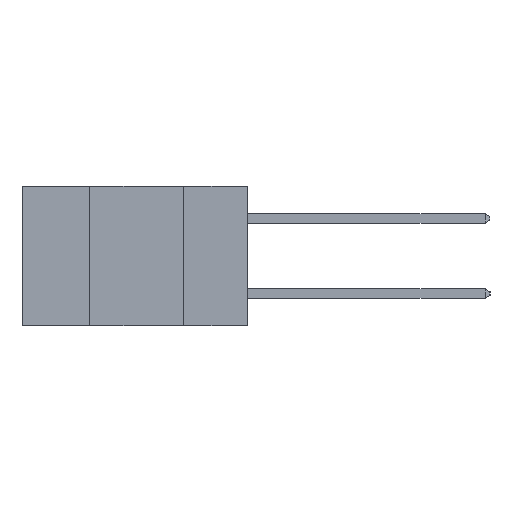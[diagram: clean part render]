
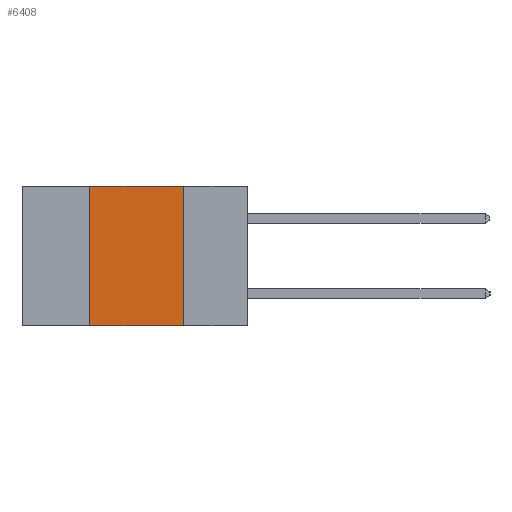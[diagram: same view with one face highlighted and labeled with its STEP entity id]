
A CAD part, left-side view. The second image highlights one B-rep face of the part: STEP entity #6408.
In plain terms, the highlighted planar face has unit normal (-1, 0, 0).
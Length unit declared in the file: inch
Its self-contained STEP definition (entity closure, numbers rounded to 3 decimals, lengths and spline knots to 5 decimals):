
#163 = DIRECTION ( 'NONE',  ( 0., -1., 0. ) ) ;
#276 = CARTESIAN_POINT ( 'NONE',  ( 0., 0.6, 0. ) ) ;
#285 = ORIENTED_EDGE ( 'NONE', *, *, #1232, .F. ) ;
#347 = VECTOR ( 'NONE', #7281, 39.37008 ) ;
#622 = DIRECTION ( 'NONE',  ( 0., 0., 1. ) ) ;
#681 = VERTEX_POINT ( 'NONE', #9778 ) ;
#891 = EDGE_LOOP ( 'NONE', ( #9026, #285, #3984, #10460 ) ) ;
#956 = LINE ( 'NONE', #11205, #10092 ) ;
#1057 = CARTESIAN_POINT ( 'NONE',  ( 0., 0.17, -0.37 ) ) ;
#1232 = EDGE_CURVE ( 'NONE', #3908, #3191, #4190, .T. ) ;
#1234 = FACE_OUTER_BOUND ( 'NONE', #891, .T. ) ;
#1329 = VERTEX_POINT ( 'NONE', #2816 ) ;
#1766 = DIRECTION ( 'NONE',  ( 0., 0., -1. ) ) ;
#2512 = EDGE_CURVE ( 'NONE', #3191, #681, #8621, .T. ) ;
#2515 = LINE ( 'NONE', #3765, #6845 ) ;
#2647 = EDGE_CURVE ( 'NONE', #1329, #681, #2515, .T. ) ;
#2704 = CARTESIAN_POINT ( 'NONE',  ( 0., 0.6, 0. ) ) ;
#2816 = CARTESIAN_POINT ( 'NONE',  ( 0., 0.42, -0.37 ) ) ;
#2960 = CARTESIAN_POINT ( 'NONE',  ( 0., 0.17, 0. ) ) ;
#3191 = VERTEX_POINT ( 'NONE', #2960 ) ;
#3552 = PLANE ( 'NONE',  #5103 ) ;
#3765 = CARTESIAN_POINT ( 'NONE',  ( 0., 0.6, -0.37 ) ) ;
#3908 = VERTEX_POINT ( 'NONE', #6883 ) ;
#3984 = ORIENTED_EDGE ( 'NONE', *, *, #6536, .F. ) ;
#4190 = LINE ( 'NONE', #276, #9193 ) ;
#5103 = AXIS2_PLACEMENT_3D ( 'NONE', #2704, #6149, #1766 ) ;
#6149 = DIRECTION ( 'NONE',  ( 1., 0., 0. ) ) ;
#6408 = ADVANCED_FACE ( 'NONE', ( #1234 ), #3552, .F. ) ;
#6509 = DIRECTION ( 'NONE',  ( 0., -1., 0. ) ) ;
#6536 = EDGE_CURVE ( 'NONE', #1329, #3908, #956, .T. ) ;
#6845 = VECTOR ( 'NONE', #163, 39.37008 ) ;
#6883 = CARTESIAN_POINT ( 'NONE',  ( 0., 0.42, 0. ) ) ;
#7281 = DIRECTION ( 'NONE',  ( 0., 0., -1. ) ) ;
#8621 = LINE ( 'NONE', #1057, #347 ) ;
#9026 = ORIENTED_EDGE ( 'NONE', *, *, #2512, .F. ) ;
#9193 = VECTOR ( 'NONE', #6509, 39.37008 ) ;
#9778 = CARTESIAN_POINT ( 'NONE',  ( 0., 0.17, -0.37 ) ) ;
#10092 = VECTOR ( 'NONE', #622, 39.37008 ) ;
#10460 = ORIENTED_EDGE ( 'NONE', *, *, #2647, .T. ) ;
#11205 = CARTESIAN_POINT ( 'NONE',  ( 0., 0.42, -0.37 ) ) ;
